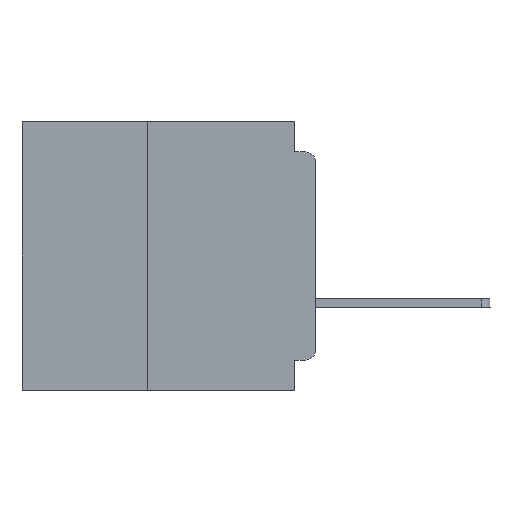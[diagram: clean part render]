
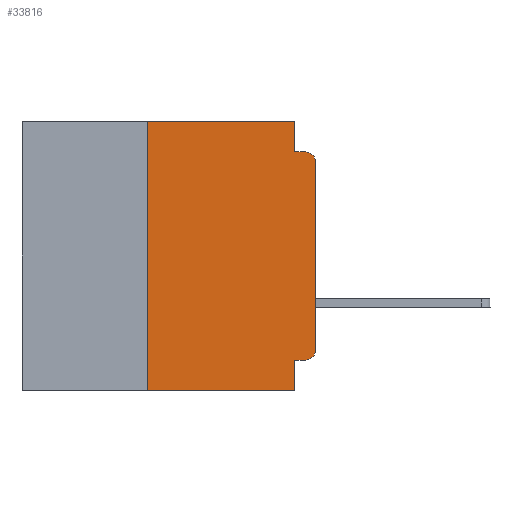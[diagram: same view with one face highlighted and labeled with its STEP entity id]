
A CAD part, left-side view. The second image highlights one B-rep face of the part: STEP entity #33816.
In plain terms, the highlighted planar face has unit normal (-1, 0, 0).
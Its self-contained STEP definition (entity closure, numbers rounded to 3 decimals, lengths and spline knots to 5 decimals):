
#1880 = CARTESIAN_POINT ( 'NONE',  ( 0., 0.015, -0.34 ) ) ;
#2467 = DIRECTION ( 'NONE',  ( 0., 1., 0. ) ) ;
#2623 = ORIENTED_EDGE ( 'NONE', *, *, #12587, .T. ) ;
#2739 = VERTEX_POINT ( 'NONE', #30491 ) ;
#2794 = EDGE_CURVE ( 'NONE', #49766, #25918, #39341, .T. ) ;
#2913 = CARTESIAN_POINT ( 'NONE',  ( 0., 0.015, -0.06 ) ) ;
#3136 = CARTESIAN_POINT ( 'NONE',  ( 0., 0., -0.06 ) ) ;
#4136 = VERTEX_POINT ( 'NONE', #58590 ) ;
#4153 = EDGE_CURVE ( 'NONE', #2739, #9699, #33657, .T. ) ;
#5293 = ORIENTED_EDGE ( 'NONE', *, *, #28487, .T. ) ;
#5350 = AXIS2_PLACEMENT_3D ( 'NONE', #54243, #39175, #8388 ) ;
#6577 = DIRECTION ( 'NONE',  ( 0., -1., 0. ) ) ;
#7002 = DIRECTION ( 'NONE',  ( 0., 0., -1. ) ) ;
#7029 = CARTESIAN_POINT ( 'NONE',  ( 0., 0., 0. ) ) ;
#7557 = DIRECTION ( 'NONE',  ( 0., -1., 0. ) ) ;
#8016 = DIRECTION ( 'NONE',  ( 0., 0., -1. ) ) ;
#8233 = ORIENTED_EDGE ( 'NONE', *, *, #26017, .F. ) ;
#8388 = DIRECTION ( 'NONE',  ( 0., 0., -1. ) ) ;
#9091 = VECTOR ( 'NONE', #7557, 39.37008 ) ;
#9699 = VERTEX_POINT ( 'NONE', #44033 ) ;
#9890 = VECTOR ( 'NONE', #2467, 39.37008 ) ;
#10020 = ORIENTED_EDGE ( 'NONE', *, *, #4153, .F. ) ;
#11278 = CARTESIAN_POINT ( 'NONE',  ( 0., 0.015, -0.045 ) ) ;
#12100 = VECTOR ( 'NONE', #64975, 39.37008 ) ;
#12360 = LINE ( 'NONE', #17727, #9091 ) ;
#12587 = EDGE_CURVE ( 'NONE', #2739, #25918, #32251, .T. ) ;
#12795 = VERTEX_POINT ( 'NONE', #28613 ) ;
#13411 = EDGE_CURVE ( 'NONE', #24503, #47140, #24222, .T. ) ;
#14377 = LINE ( 'NONE', #7029, #40030 ) ;
#16476 = VERTEX_POINT ( 'NONE', #18521 ) ;
#17727 = CARTESIAN_POINT ( 'NONE',  ( 0., 0., -0.045 ) ) ;
#18058 = DIRECTION ( 'NONE',  ( 0., 0., 1. ) ) ;
#18521 = CARTESIAN_POINT ( 'NONE',  ( 0., 0.015, -0.355 ) ) ;
#18613 = VECTOR ( 'NONE', #6577, 39.37008 ) ;
#18994 = VERTEX_POINT ( 'NONE', #48337 ) ;
#20613 = DIRECTION ( 'NONE',  ( 0., 0., -1. ) ) ;
#21408 = EDGE_CURVE ( 'NONE', #4136, #12795, #39400, .T. ) ;
#21766 = ORIENTED_EDGE ( 'NONE', *, *, #21408, .F. ) ;
#21835 = DIRECTION ( 'NONE',  ( 0., -1., 0. ) ) ;
#23023 = FACE_OUTER_BOUND ( 'NONE', #61903, .T. ) ;
#23514 = ORIENTED_EDGE ( 'NONE', *, *, #13411, .T. ) ;
#24222 = CIRCLE ( 'NONE', #65529, 0.015 ) ;
#24503 = VERTEX_POINT ( 'NONE', #3136 ) ;
#25345 = AXIS2_PLACEMENT_3D ( 'NONE', #1880, #37793, #7002 ) ;
#25539 = ORIENTED_EDGE ( 'NONE', *, *, #63394, .F. ) ;
#25918 = VERTEX_POINT ( 'NONE', #51476 ) ;
#26017 = EDGE_CURVE ( 'NONE', #9699, #4136, #41828, .T. ) ;
#26835 = LINE ( 'NONE', #63623, #9890 ) ;
#28263 = VECTOR ( 'NONE', #21835, 39.37008 ) ;
#28487 = EDGE_CURVE ( 'NONE', #16476, #18994, #62887, .T. ) ;
#28613 = CARTESIAN_POINT ( 'NONE',  ( 0., 0.031, -0.045 ) ) ;
#28900 = PLANE ( 'NONE',  #5350 ) ;
#30491 = CARTESIAN_POINT ( 'NONE',  ( 0., 0.25, -0.4 ) ) ;
#30706 = CARTESIAN_POINT ( 'NONE',  ( 0., 0.031, -0.4 ) ) ;
#32251 = LINE ( 'NONE', #37362, #18613 ) ;
#33657 = LINE ( 'NONE', #48387, #43990 ) ;
#33816 = ADVANCED_FACE ( 'NONE', ( #23023 ), #28900, .F. ) ;
#37362 = CARTESIAN_POINT ( 'NONE',  ( 0., 0.437, -0.4 ) ) ;
#37503 = EDGE_CURVE ( 'NONE', #16476, #49766, #26835, .T. ) ;
#37793 = DIRECTION ( 'NONE',  ( -1., 0., 0. ) ) ;
#38826 = DIRECTION ( 'NONE',  ( -1., 0., 0. ) ) ;
#39175 = DIRECTION ( 'NONE',  ( 1., 0., 0. ) ) ;
#39341 = LINE ( 'NONE', #30706, #64698 ) ;
#39400 = LINE ( 'NONE', #44579, #12100 ) ;
#40030 = VECTOR ( 'NONE', #53095, 39.37008 ) ;
#41828 = LINE ( 'NONE', #57432, #28263 ) ;
#43990 = VECTOR ( 'NONE', #18058, 39.37008 ) ;
#44033 = CARTESIAN_POINT ( 'NONE',  ( 0., 0.25, 0. ) ) ;
#44579 = CARTESIAN_POINT ( 'NONE',  ( 0., 0.031, 0. ) ) ;
#47140 = VERTEX_POINT ( 'NONE', #11278 ) ;
#48337 = CARTESIAN_POINT ( 'NONE',  ( 0., 0., -0.34 ) ) ;
#48387 = CARTESIAN_POINT ( 'NONE',  ( 0., 0.25, -0.4 ) ) ;
#49766 = VERTEX_POINT ( 'NONE', #63410 ) ;
#51476 = CARTESIAN_POINT ( 'NONE',  ( 0., 0.031, -0.4 ) ) ;
#51715 = ORIENTED_EDGE ( 'NONE', *, *, #2794, .F. ) ;
#52979 = ORIENTED_EDGE ( 'NONE', *, *, #54096, .T. ) ;
#53095 = DIRECTION ( 'NONE',  ( 0., 0., 1. ) ) ;
#53529 = ORIENTED_EDGE ( 'NONE', *, *, #37503, .F. ) ;
#54096 = EDGE_CURVE ( 'NONE', #18994, #24503, #14377, .T. ) ;
#54243 = CARTESIAN_POINT ( 'NONE',  ( 0., 0.437, 0. ) ) ;
#57432 = CARTESIAN_POINT ( 'NONE',  ( 0., 0.437, 0. ) ) ;
#58590 = CARTESIAN_POINT ( 'NONE',  ( 0., 0.031, 0. ) ) ;
#61903 = EDGE_LOOP ( 'NONE', ( #52979, #23514, #25539, #21766, #8233, #10020, #2623, #51715, #53529, #5293 ) ) ;
#62887 = CIRCLE ( 'NONE', #25345, 0.015 ) ;
#63394 = EDGE_CURVE ( 'NONE', #12795, #47140, #12360, .T. ) ;
#63410 = CARTESIAN_POINT ( 'NONE',  ( 0., 0.031, -0.355 ) ) ;
#63623 = CARTESIAN_POINT ( 'NONE',  ( 0., 0., -0.355 ) ) ;
#64698 = VECTOR ( 'NONE', #20613, 39.37008 ) ;
#64975 = DIRECTION ( 'NONE',  ( 0., 0., -1. ) ) ;
#65529 = AXIS2_PLACEMENT_3D ( 'NONE', #2913, #38826, #8016 ) ;
